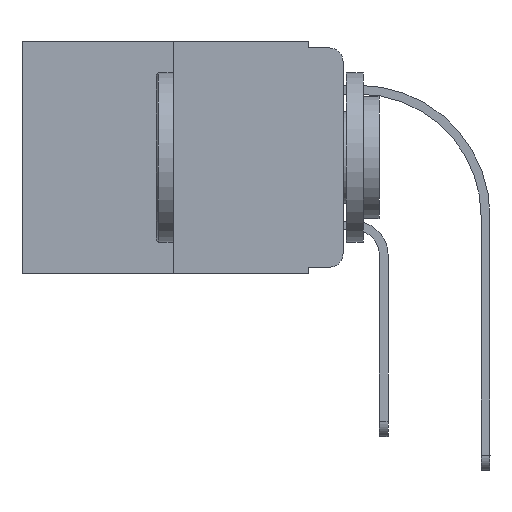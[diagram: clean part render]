
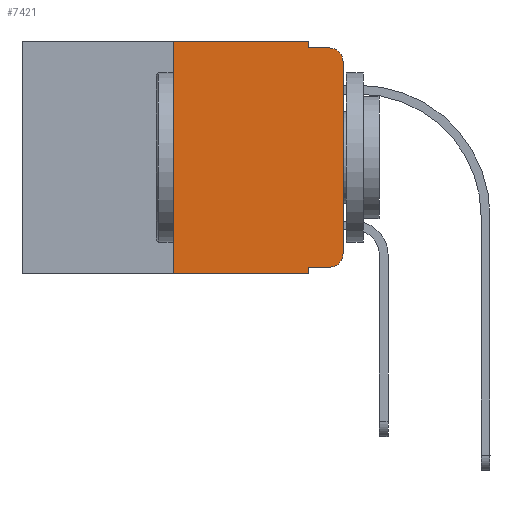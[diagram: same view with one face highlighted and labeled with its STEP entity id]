
A CAD part, left-side view. The second image highlights one B-rep face of the part: STEP entity #7421.
In plain terms, the highlighted planar face has unit normal (-1, 0, 0).
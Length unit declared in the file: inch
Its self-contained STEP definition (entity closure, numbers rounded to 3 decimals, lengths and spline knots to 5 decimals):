
#133 = EDGE_CURVE ( 'NONE', #13715, #6347, #5046, .T. ) ;
#193 = CARTESIAN_POINT ( 'NONE',  ( 0., 0., -0.313 ) ) ;
#245 = DIRECTION ( 'NONE',  ( 0., -1., 0. ) ) ;
#266 = EDGE_LOOP ( 'NONE', ( #4135, #11167, #9972, #14454, #5539, #11950, #3955, #5636, #7934, #11509 ) ) ;
#379 = DIRECTION ( 'NONE',  ( 0., 0., 1. ) ) ;
#451 = VECTOR ( 'NONE', #379, 39.37008 ) ;
#650 = FACE_OUTER_BOUND ( 'NONE', #266, .T. ) ;
#842 = CARTESIAN_POINT ( 'NONE',  ( 0., 0.051, -0.343 ) ) ;
#974 = EDGE_CURVE ( 'NONE', #6482, #5798, #6078, .T. ) ;
#1083 = DIRECTION ( 'NONE',  ( 0., -1., 0. ) ) ;
#1128 = AXIS2_PLACEMENT_3D ( 'NONE', #6949, #11770, #8092 ) ;
#1212 = VERTEX_POINT ( 'NONE', #6801 ) ;
#1942 = VERTEX_POINT ( 'NONE', #3796 ) ;
#2168 = LINE ( 'NONE', #10901, #10671 ) ;
#2247 = DIRECTION ( 'NONE',  ( 0., 0., -1. ) ) ;
#2295 = CARTESIAN_POINT ( 'NONE',  ( 0., 0.02, -0.01 ) ) ;
#2463 = CARTESIAN_POINT ( 'NONE',  ( 0., 0.473, -0.343 ) ) ;
#2501 = VERTEX_POINT ( 'NONE', #11783 ) ;
#2843 = VECTOR ( 'NONE', #245, 39.37008 ) ;
#3273 = VERTEX_POINT ( 'NONE', #5214 ) ;
#3346 = VERTEX_POINT ( 'NONE', #842 ) ;
#3796 = CARTESIAN_POINT ( 'NONE',  ( 0., 0., -0.03 ) ) ;
#3874 = LINE ( 'NONE', #13435, #5192 ) ;
#3931 = CARTESIAN_POINT ( 'NONE',  ( 0., 0.051, -0.333 ) ) ;
#3955 = ORIENTED_EDGE ( 'NONE', *, *, #5879, .T. ) ;
#4092 = DIRECTION ( 'NONE',  ( 0., 0., -1. ) ) ;
#4135 = ORIENTED_EDGE ( 'NONE', *, *, #9650, .T. ) ;
#4222 = CARTESIAN_POINT ( 'NONE',  ( 0., 0.051, 0. ) ) ;
#4270 = DIRECTION ( 'NONE',  ( 0., 0., -1. ) ) ;
#4370 = CARTESIAN_POINT ( 'NONE',  ( 0., 0.473, 0. ) ) ;
#5046 = LINE ( 'NONE', #9045, #451 ) ;
#5192 = VECTOR ( 'NONE', #2247, 39.37008 ) ;
#5214 = CARTESIAN_POINT ( 'NONE',  ( 0., 0.051, 0. ) ) ;
#5238 = EDGE_CURVE ( 'NONE', #6347, #3273, #10742, .T. ) ;
#5239 = CIRCLE ( 'NONE', #11998, 0.02 ) ;
#5539 = ORIENTED_EDGE ( 'NONE', *, *, #5238, .F. ) ;
#5564 = PLANE ( 'NONE',  #1128 ) ;
#5610 = DIRECTION ( 'NONE',  ( 0., 0., -1. ) ) ;
#5636 = ORIENTED_EDGE ( 'NONE', *, *, #9869, .F. ) ;
#5648 = DIRECTION ( 'NONE',  ( -1., 0., 0. ) ) ;
#5798 = VERTEX_POINT ( 'NONE', #2295 ) ;
#5879 = EDGE_CURVE ( 'NONE', #13715, #3346, #13640, .T. ) ;
#6078 = LINE ( 'NONE', #12277, #12845 ) ;
#6223 = CARTESIAN_POINT ( 'NONE',  ( 0., 0.02, -0.03 ) ) ;
#6347 = VERTEX_POINT ( 'NONE', #13385 ) ;
#6473 = CIRCLE ( 'NONE', #15068, 0.02 ) ;
#6482 = VERTEX_POINT ( 'NONE', #13696 ) ;
#6801 = CARTESIAN_POINT ( 'NONE',  ( 0., 0.051, -0.333 ) ) ;
#6949 = CARTESIAN_POINT ( 'NONE',  ( 0., 0.473, 0. ) ) ;
#7421 = ADVANCED_FACE ( 'NONE', ( #650 ), #5564, .F. ) ;
#7675 = VECTOR ( 'NONE', #12421, 39.37008 ) ;
#7934 = ORIENTED_EDGE ( 'NONE', *, *, #13213, .T. ) ;
#8092 = DIRECTION ( 'NONE',  ( 0., 0., -1. ) ) ;
#8200 = EDGE_CURVE ( 'NONE', #3273, #6482, #15553, .T. ) ;
#9045 = CARTESIAN_POINT ( 'NONE',  ( 0., 0.25, 0. ) ) ;
#9650 = EDGE_CURVE ( 'NONE', #11252, #1942, #2168, .T. ) ;
#9869 = EDGE_CURVE ( 'NONE', #1212, #3346, #3874, .T. ) ;
#9972 = ORIENTED_EDGE ( 'NONE', *, *, #974, .F. ) ;
#10507 = EDGE_CURVE ( 'NONE', #2501, #11252, #6473, .T. ) ;
#10671 = VECTOR ( 'NONE', #10751, 39.37008 ) ;
#10742 = LINE ( 'NONE', #4370, #12559 ) ;
#10751 = DIRECTION ( 'NONE',  ( 0., 0., 1. ) ) ;
#10901 = CARTESIAN_POINT ( 'NONE',  ( 0., 0., 0. ) ) ;
#11167 = ORIENTED_EDGE ( 'NONE', *, *, #14528, .T. ) ;
#11252 = VERTEX_POINT ( 'NONE', #193 ) ;
#11509 = ORIENTED_EDGE ( 'NONE', *, *, #10507, .T. ) ;
#11770 = DIRECTION ( 'NONE',  ( 1., 0., 0. ) ) ;
#11783 = CARTESIAN_POINT ( 'NONE',  ( 0., 0.02, -0.333 ) ) ;
#11950 = ORIENTED_EDGE ( 'NONE', *, *, #133, .F. ) ;
#11998 = AXIS2_PLACEMENT_3D ( 'NONE', #6223, #12425, #4092 ) ;
#12277 = CARTESIAN_POINT ( 'NONE',  ( 0., 0.051, -0.01 ) ) ;
#12421 = DIRECTION ( 'NONE',  ( 0., -1., 0. ) ) ;
#12425 = DIRECTION ( 'NONE',  ( -1., 0., 0. ) ) ;
#12559 = VECTOR ( 'NONE', #14557, 39.37008 ) ;
#12845 = VECTOR ( 'NONE', #1083, 39.37008 ) ;
#13213 = EDGE_CURVE ( 'NONE', #1212, #2501, #16078, .T. ) ;
#13308 = CARTESIAN_POINT ( 'NONE',  ( 0., 0.02, -0.313 ) ) ;
#13385 = CARTESIAN_POINT ( 'NONE',  ( 0., 0.25, 0. ) ) ;
#13435 = CARTESIAN_POINT ( 'NONE',  ( 0., 0.051, 0. ) ) ;
#13640 = LINE ( 'NONE', #2463, #7675 ) ;
#13696 = CARTESIAN_POINT ( 'NONE',  ( 0., 0.051, -0.01 ) ) ;
#13715 = VERTEX_POINT ( 'NONE', #13759 ) ;
#13759 = CARTESIAN_POINT ( 'NONE',  ( 0., 0.25, -0.343 ) ) ;
#13895 = VECTOR ( 'NONE', #5610, 39.37008 ) ;
#14454 = ORIENTED_EDGE ( 'NONE', *, *, #8200, .F. ) ;
#14528 = EDGE_CURVE ( 'NONE', #1942, #5798, #5239, .T. ) ;
#14557 = DIRECTION ( 'NONE',  ( 0., -1., 0. ) ) ;
#15068 = AXIS2_PLACEMENT_3D ( 'NONE', #13308, #5648, #4270 ) ;
#15553 = LINE ( 'NONE', #4222, #13895 ) ;
#16078 = LINE ( 'NONE', #3931, #2843 ) ;
